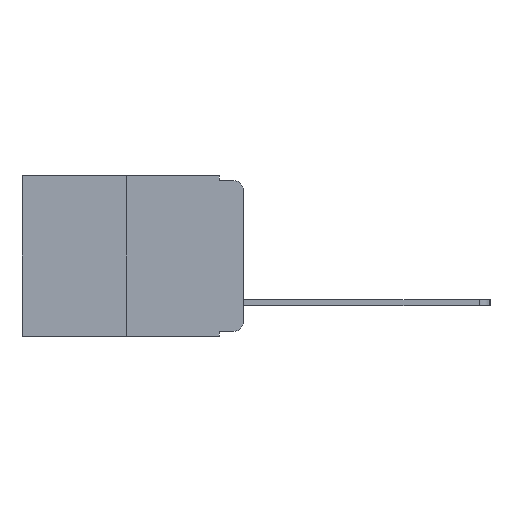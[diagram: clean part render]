
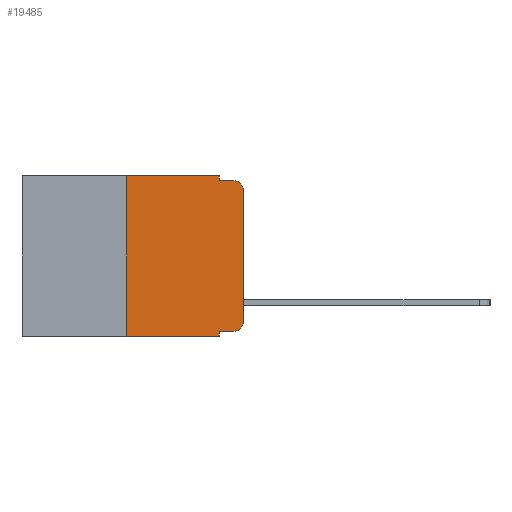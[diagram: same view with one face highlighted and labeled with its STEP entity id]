
A CAD part, left-side view. The second image highlights one B-rep face of the part: STEP entity #19485.
In plain terms, the highlighted planar face has unit normal (-1, 0, 0).
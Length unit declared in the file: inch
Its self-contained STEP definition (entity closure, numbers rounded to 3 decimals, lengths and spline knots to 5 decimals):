
#953 = EDGE_CURVE ( 'NONE', #8773, #6973, #15762, .T. ) ;
#2080 = ORIENTED_EDGE ( 'NONE', *, *, #15423, .T. ) ;
#2166 = ORIENTED_EDGE ( 'NONE', *, *, #5585, .T. ) ;
#2178 = DIRECTION ( 'NONE',  ( 1., 0., 0. ) ) ;
#2197 = CARTESIAN_POINT ( 'NONE',  ( 0., 0.02, -0.01 ) ) ;
#2238 = VECTOR ( 'NONE', #17603, 39.37008 ) ;
#2464 = ORIENTED_EDGE ( 'NONE', *, *, #953, .F. ) ;
#2539 = LINE ( 'NONE', #15790, #19703 ) ;
#2731 = CARTESIAN_POINT ( 'NONE',  ( 0., 0.051, -0.343 ) ) ;
#2859 = ORIENTED_EDGE ( 'NONE', *, *, #8294, .F. ) ;
#2929 = CARTESIAN_POINT ( 'NONE',  ( 0., 0.02, -0.03 ) ) ;
#3006 = EDGE_CURVE ( 'NONE', #8052, #10826, #2539, .T. ) ;
#3013 = EDGE_LOOP ( 'NONE', ( #2080, #2166, #2464, #2859, #3126, #3168, #3942, #4003, #4220, #4263 ) ) ;
#3126 = ORIENTED_EDGE ( 'NONE', *, *, #17642, .F. ) ;
#3168 = ORIENTED_EDGE ( 'NONE', *, *, #3006, .F. ) ;
#3347 = LINE ( 'NONE', #16881, #11786 ) ;
#3840 = DIRECTION ( 'NONE',  ( 0., -1., 0. ) ) ;
#3942 = ORIENTED_EDGE ( 'NONE', *, *, #14537, .T. ) ;
#4003 = ORIENTED_EDGE ( 'NONE', *, *, #4570, .F. ) ;
#4130 = CARTESIAN_POINT ( 'NONE',  ( 0., 0.051, -0.333 ) ) ;
#4220 = ORIENTED_EDGE ( 'NONE', *, *, #12169, .T. ) ;
#4263 = ORIENTED_EDGE ( 'NONE', *, *, #18703, .T. ) ;
#4570 = EDGE_CURVE ( 'NONE', #7902, #18577, #19425, .T. ) ;
#4643 = DIRECTION ( 'NONE',  ( 0., 0., -1. ) ) ;
#4675 = CARTESIAN_POINT ( 'NONE',  ( 0., 0., -0.03 ) ) ;
#5135 = DIRECTION ( 'NONE',  ( -1., 0., 0. ) ) ;
#5226 = DIRECTION ( 'NONE',  ( 0., -1., 0. ) ) ;
#5360 = VECTOR ( 'NONE', #7139, 39.37008 ) ;
#5536 = CARTESIAN_POINT ( 'NONE',  ( 0., 0.473, 0. ) ) ;
#5552 = DIRECTION ( 'NONE',  ( 0., 0., 1. ) ) ;
#5585 = EDGE_CURVE ( 'NONE', #10554, #6973, #8054, .T. ) ;
#5827 = DIRECTION ( 'NONE',  ( 0., -1., 0. ) ) ;
#5875 = LINE ( 'NONE', #8848, #5360 ) ;
#6042 = DIRECTION ( 'NONE',  ( 0., 0., 1. ) ) ;
#6555 = CARTESIAN_POINT ( 'NONE',  ( 0., 0.02, -0.333 ) ) ;
#6692 = VECTOR ( 'NONE', #5827, 39.37008 ) ;
#6973 = VERTEX_POINT ( 'NONE', #2197 ) ;
#7095 = VECTOR ( 'NONE', #16709, 39.37008 ) ;
#7139 = DIRECTION ( 'NONE',  ( 0., -1., 0. ) ) ;
#7550 = VERTEX_POINT ( 'NONE', #6555 ) ;
#7902 = VERTEX_POINT ( 'NONE', #18694 ) ;
#8052 = VERTEX_POINT ( 'NONE', #12963 ) ;
#8054 = CIRCLE ( 'NONE', #9409, 0.02 ) ;
#8294 = EDGE_CURVE ( 'NONE', #8422, #8773, #17624, .T. ) ;
#8422 = VERTEX_POINT ( 'NONE', #12318 ) ;
#8773 = VERTEX_POINT ( 'NONE', #10159 ) ;
#8848 = CARTESIAN_POINT ( 'NONE',  ( 0., 0.473, 0. ) ) ;
#9409 = AXIS2_PLACEMENT_3D ( 'NONE', #2929, #14507, #4643 ) ;
#10045 = CARTESIAN_POINT ( 'NONE',  ( 0., 0., -0.313 ) ) ;
#10159 = CARTESIAN_POINT ( 'NONE',  ( 0., 0.051, -0.01 ) ) ;
#10554 = VERTEX_POINT ( 'NONE', #4675 ) ;
#10826 = VERTEX_POINT ( 'NONE', #15323 ) ;
#11638 = VECTOR ( 'NONE', #3840, 39.37008 ) ;
#11786 = VECTOR ( 'NONE', #5552, 39.37008 ) ;
#11918 = CARTESIAN_POINT ( 'NONE',  ( 0., 0.051, -0.01 ) ) ;
#12169 = EDGE_CURVE ( 'NONE', #7902, #7550, #19859, .T. ) ;
#12318 = CARTESIAN_POINT ( 'NONE',  ( 0., 0.051, 0. ) ) ;
#12383 = CIRCLE ( 'NONE', #19026, 0.02 ) ;
#12963 = CARTESIAN_POINT ( 'NONE',  ( 0., 0.25, -0.343 ) ) ;
#13054 = CARTESIAN_POINT ( 'NONE',  ( 0., 0.051, 0. ) ) ;
#13492 = CARTESIAN_POINT ( 'NONE',  ( 0., 0.473, -0.343 ) ) ;
#13849 = DIRECTION ( 'NONE',  ( 0., 0., -1. ) ) ;
#14507 = DIRECTION ( 'NONE',  ( -1., 0., 0. ) ) ;
#14537 = EDGE_CURVE ( 'NONE', #8052, #18577, #20000, .T. ) ;
#14842 = AXIS2_PLACEMENT_3D ( 'NONE', #5536, #2178, #13849 ) ;
#14941 = CARTESIAN_POINT ( 'NONE',  ( 0., 0.02, -0.313 ) ) ;
#15160 = CARTESIAN_POINT ( 'NONE',  ( 0., 0.051, 0. ) ) ;
#15247 = PLANE ( 'NONE',  #14842 ) ;
#15323 = CARTESIAN_POINT ( 'NONE',  ( 0., 0.25, 0. ) ) ;
#15423 = EDGE_CURVE ( 'NONE', #20778, #10554, #3347, .T. ) ;
#15762 = LINE ( 'NONE', #11918, #11638 ) ;
#15790 = CARTESIAN_POINT ( 'NONE',  ( 0., 0.25, 0. ) ) ;
#16497 = DIRECTION ( 'NONE',  ( 0., 0., -1. ) ) ;
#16709 = DIRECTION ( 'NONE',  ( 0., 0., -1. ) ) ;
#16881 = CARTESIAN_POINT ( 'NONE',  ( 0., 0., 0. ) ) ;
#17603 = DIRECTION ( 'NONE',  ( 0., 0., -1. ) ) ;
#17624 = LINE ( 'NONE', #15160, #7095 ) ;
#17642 = EDGE_CURVE ( 'NONE', #10826, #8422, #5875, .T. ) ;
#18577 = VERTEX_POINT ( 'NONE', #2731 ) ;
#18694 = CARTESIAN_POINT ( 'NONE',  ( 0., 0.051, -0.333 ) ) ;
#18703 = EDGE_CURVE ( 'NONE', #7550, #20778, #12383, .T. ) ;
#19026 = AXIS2_PLACEMENT_3D ( 'NONE', #14941, #5135, #16497 ) ;
#19238 = VECTOR ( 'NONE', #5226, 39.37008 ) ;
#19425 = LINE ( 'NONE', #13054, #2238 ) ;
#19485 = ADVANCED_FACE ( 'NONE', ( #20492 ), #15247, .F. ) ;
#19703 = VECTOR ( 'NONE', #6042, 39.37008 ) ;
#19859 = LINE ( 'NONE', #4130, #6692 ) ;
#20000 = LINE ( 'NONE', #13492, #19238 ) ;
#20492 = FACE_OUTER_BOUND ( 'NONE', #3013, .T. ) ;
#20778 = VERTEX_POINT ( 'NONE', #10045 ) ;
